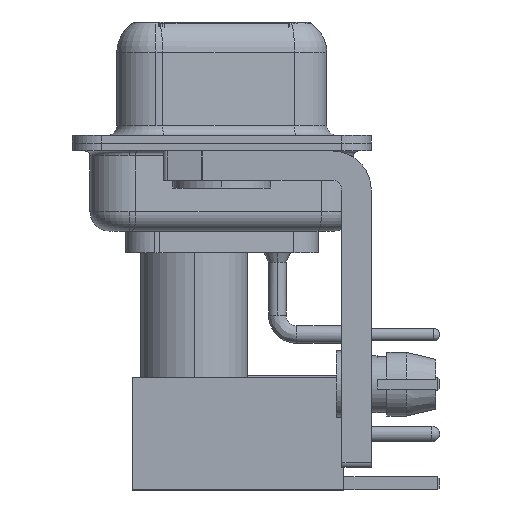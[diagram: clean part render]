
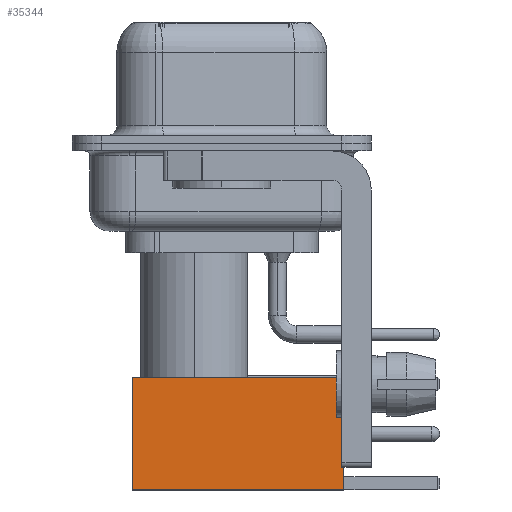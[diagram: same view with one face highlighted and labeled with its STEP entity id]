
A CAD part, left-side view. The second image highlights one B-rep face of the part: STEP entity #35344.
In plain terms, the highlighted face is planar.
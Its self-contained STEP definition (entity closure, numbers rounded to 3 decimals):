
#138 = VECTOR ( 'NONE', #28832, 1000. ) ;
#346 = EDGE_CURVE ( 'NONE', #2418, #32188, #7264, .T. ) ;
#1795 = CARTESIAN_POINT ( 'NONE',  ( 0., 2.875, 10.82 ) ) ;
#2056 = DIRECTION ( 'NONE',  ( -1., 0., 0. ) ) ;
#2418 = VERTEX_POINT ( 'NONE', #2460 ) ;
#2460 = CARTESIAN_POINT ( 'NONE',  ( 2.875, 2.875, 10.82 ) ) ;
#3400 = FACE_OUTER_BOUND ( 'NONE', #31505, .T. ) ;
#5130 = EDGE_CURVE ( 'NONE', #19243, #28547, #26722, .T. ) ;
#7184 = ORIENTED_EDGE ( 'NONE', *, *, #5130, .F. ) ;
#7264 = LINE ( 'NONE', #31821, #138 ) ;
#9233 = ORIENTED_EDGE ( 'NONE', *, *, #21662, .T. ) ;
#10757 = EDGE_CURVE ( 'NONE', #2418, #19243, #14553, .T. ) ;
#12324 = CARTESIAN_POINT ( 'NONE',  ( -2.875, 2.875, 0. ) ) ;
#14553 = LINE ( 'NONE', #1795, #31007 ) ;
#15768 = CARTESIAN_POINT ( 'NONE',  ( 2.875, 2.875, 0. ) ) ;
#16956 = DIRECTION ( 'NONE',  ( -1., 0., 0. ) ) ;
#19243 = VERTEX_POINT ( 'NONE', #28896 ) ;
#19734 = ORIENTED_EDGE ( 'NONE', *, *, #346, .T. ) ;
#20333 = CARTESIAN_POINT ( 'NONE',  ( 2.875, 2.875, 0. ) ) ;
#20578 = VECTOR ( 'NONE', #29127, 1000. ) ;
#20987 = CARTESIAN_POINT ( 'NONE',  ( 0., 2.875, 0. ) ) ;
#21662 = EDGE_CURVE ( 'NONE', #32188, #28547, #29788, .T. ) ;
#25845 = ORIENTED_EDGE ( 'NONE', *, *, #10757, .F. ) ;
#26700 = AXIS2_PLACEMENT_3D ( 'NONE', #15768, #33753, #36948 ) ;
#26722 = LINE ( 'NONE', #32524, #20578 ) ;
#28547 = VERTEX_POINT ( 'NONE', #12324 ) ;
#28832 = DIRECTION ( 'NONE',  ( 0., 0., -1. ) ) ;
#28896 = CARTESIAN_POINT ( 'NONE',  ( -2.875, 2.875, 10.82 ) ) ;
#29127 = DIRECTION ( 'NONE',  ( 0., 0., -1. ) ) ;
#29788 = LINE ( 'NONE', #20987, #37566 ) ;
#31007 = VECTOR ( 'NONE', #16956, 1000. ) ;
#31505 = EDGE_LOOP ( 'NONE', ( #19734, #9233, #7184, #25845 ) ) ;
#31821 = CARTESIAN_POINT ( 'NONE',  ( 2.875, 2.875, 0. ) ) ;
#32188 = VERTEX_POINT ( 'NONE', #20333 ) ;
#32524 = CARTESIAN_POINT ( 'NONE',  ( -2.875, 2.875, 0. ) ) ;
#33753 = DIRECTION ( 'NONE',  ( 0., 1., 0. ) ) ;
#35344 = ADVANCED_FACE ( 'NONE', ( #3400 ), #36750, .T. ) ;
#36750 = PLANE ( 'NONE',  #26700 ) ;
#36948 = DIRECTION ( 'NONE',  ( 0., 0., 1. ) ) ;
#37566 = VECTOR ( 'NONE', #2056, 1000. ) ;
